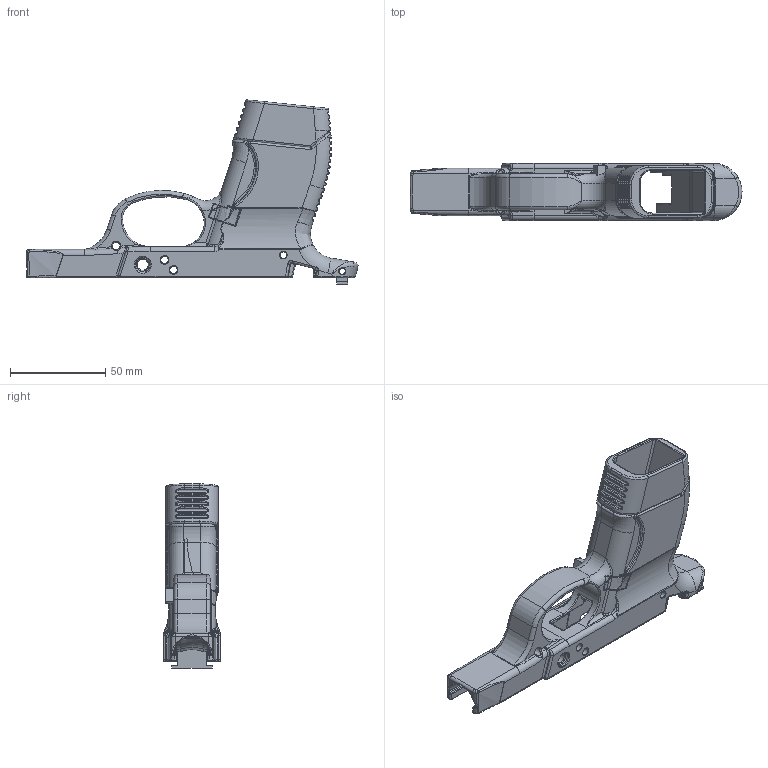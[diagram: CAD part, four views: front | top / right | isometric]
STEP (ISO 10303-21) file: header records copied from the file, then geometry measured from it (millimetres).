
FILE_DESCRIPTION(/* description */ (''),/* implementation_level */ '2;1');
FILE_NAME(/* name */ 'SR9SC.step',/* time_stamp */ '2019-11-17T18:05:57-05:00',/* author */ (''),/* organization */ (''),/* preprocessor_version */ 'ST-DEVELOPER v18',/* originating_system */ 'Autodesk Translation Framework v8.12.0.6',/* authorisation */ '');
FILE_SCHEMA (('AUTOMOTIVE_DESIGN { 1 0 10303 214 3 1 1 }'));
Products named in the file (4): SR9C G26 GRIP LENGTH; Mag Catch SR9; SR9 Rear Rail; G19 Mag Grip
Assembly tree (3 placements, depth 2):
  SR9C G26 GRIP LENGTH
    Mag Catch SR9
    SR9 Rear Rail
    G19 Mag Grip
Bounding box: 174.67 x 30 x 96.93 mm (x, y, z)
Volume: 71777.7 mm3; surface area: 44894.7 mm2
Topology: 7 solids, 7 shells, 1704 faces, 4048 edges, 2262 vertices
Faces by surface type: bspline 596, cylinder 573, plane 255, torus 207, sphere 44, cone 29
Full cylindrical faces by diameter (mm): 3.175 x3, 3.5 x1, 4 x6, 4.36 x1, 5.8 x2, 8 x1
Entity records: 66985 total; most frequent: CARTESIAN_POINT 30486, ORIENTED_EDGE 7938, DIRECTION 7192, EDGE_CURVE 3969, AXIS2_PLACEMENT_3D 2972, VERTEX_POINT 2264, EDGE_LOOP 1727, FACE_OUTER_BOUND 1704
